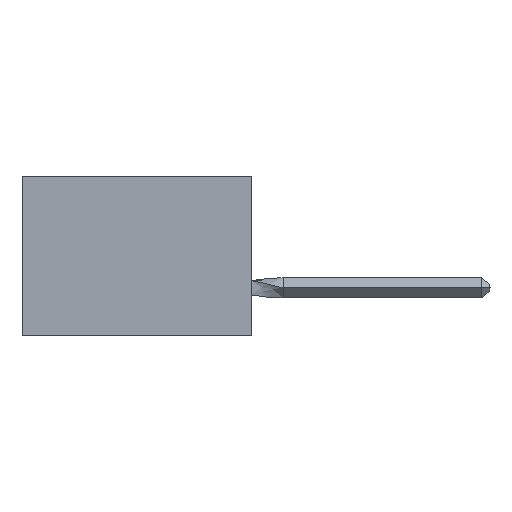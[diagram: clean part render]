
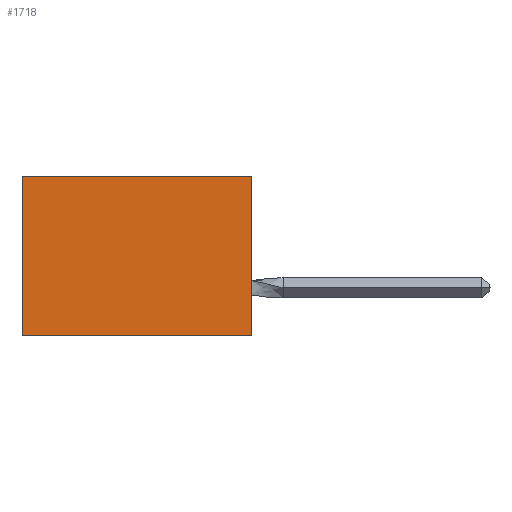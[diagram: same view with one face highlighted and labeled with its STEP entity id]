
A CAD part, left-side view. The second image highlights one B-rep face of the part: STEP entity #1718.
In plain terms, the highlighted planar face has unit normal (-1, 0, 0).
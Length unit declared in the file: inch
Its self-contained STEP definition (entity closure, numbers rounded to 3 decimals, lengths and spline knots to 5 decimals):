
#625 = ORIENTED_EDGE ( 'NONE', *, *, #7288, .F. ) ;
#1249 = CARTESIAN_POINT ( 'NONE',  ( 0.305, 0.72, -0.5 ) ) ;
#1718 = ADVANCED_FACE ( 'NONE', ( #25129 ), #6414, .F. ) ;
#2276 = CARTESIAN_POINT ( 'NONE',  ( 0.305, 0., 0. ) ) ;
#2544 = VECTOR ( 'NONE', #8706, 39.37008 ) ;
#2565 = ORIENTED_EDGE ( 'NONE', *, *, #21413, .T. ) ;
#6394 = ORIENTED_EDGE ( 'NONE', *, *, #9884, .F. ) ;
#6414 = PLANE ( 'NONE',  #9318 ) ;
#6427 = DIRECTION ( 'NONE',  ( 0., 0., -1. ) ) ;
#6432 = CARTESIAN_POINT ( 'NONE',  ( 0.305, 0., -0.5 ) ) ;
#7288 = EDGE_CURVE ( 'NONE', #9996, #14354, #16204, .T. ) ;
#7635 = ORIENTED_EDGE ( 'NONE', *, *, #14224, .T. ) ;
#8352 = CARTESIAN_POINT ( 'NONE',  ( 0.305, 0., -0.5 ) ) ;
#8425 = CARTESIAN_POINT ( 'NONE',  ( 0.305, 0., -0.5 ) ) ;
#8706 = DIRECTION ( 'NONE',  ( 0., 1., 0. ) ) ;
#8855 = VERTEX_POINT ( 'NONE', #9925 ) ;
#9318 = AXIS2_PLACEMENT_3D ( 'NONE', #8425, #10463, #12770 ) ;
#9884 = EDGE_CURVE ( 'NONE', #14354, #19068, #10422, .T. ) ;
#9925 = CARTESIAN_POINT ( 'NONE',  ( 0.305, 0.72, 0. ) ) ;
#9996 = VERTEX_POINT ( 'NONE', #2276 ) ;
#10366 = DIRECTION ( 'NONE',  ( 0., 0., -1. ) ) ;
#10422 = LINE ( 'NONE', #6432, #2544 ) ;
#10463 = DIRECTION ( 'NONE',  ( 1., 0., 0. ) ) ;
#10775 = LINE ( 'NONE', #14862, #21837 ) ;
#10826 = CARTESIAN_POINT ( 'NONE',  ( 0.305, 0., -0.5 ) ) ;
#12770 = DIRECTION ( 'NONE',  ( 0., 0., -1. ) ) ;
#14224 = EDGE_CURVE ( 'NONE', #8855, #19068, #24425, .T. ) ;
#14354 = VERTEX_POINT ( 'NONE', #10826 ) ;
#14597 = DIRECTION ( 'NONE',  ( 0., 1., 0. ) ) ;
#14862 = CARTESIAN_POINT ( 'NONE',  ( 0.305, 0., 0. ) ) ;
#16204 = LINE ( 'NONE', #8352, #17786 ) ;
#17786 = VECTOR ( 'NONE', #10366, 39.37008 ) ;
#18498 = CARTESIAN_POINT ( 'NONE',  ( 0.305, 0.72, -0.5 ) ) ;
#19068 = VERTEX_POINT ( 'NONE', #1249 ) ;
#21413 = EDGE_CURVE ( 'NONE', #9996, #8855, #10775, .T. ) ;
#21837 = VECTOR ( 'NONE', #14597, 39.37008 ) ;
#23810 = VECTOR ( 'NONE', #6427, 39.37008 ) ;
#24425 = LINE ( 'NONE', #18498, #23810 ) ;
#25129 = FACE_OUTER_BOUND ( 'NONE', #25179, .T. ) ;
#25179 = EDGE_LOOP ( 'NONE', ( #7635, #6394, #625, #2565 ) ) ;
